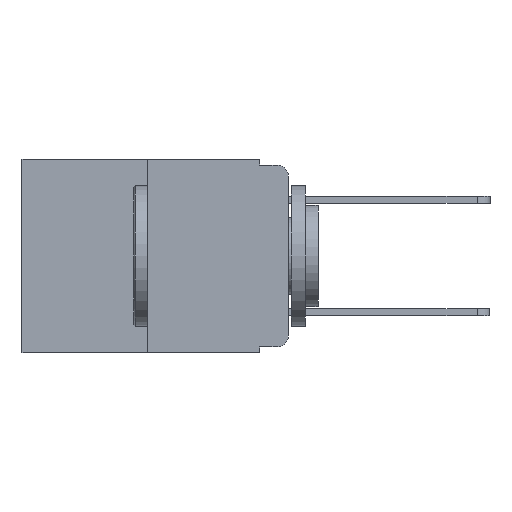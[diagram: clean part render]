
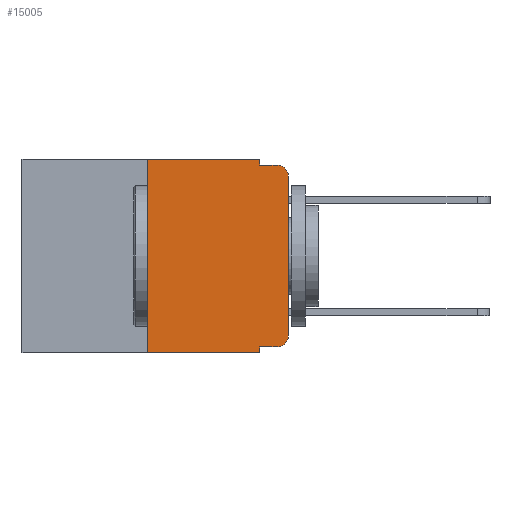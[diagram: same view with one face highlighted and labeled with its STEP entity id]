
A CAD part, left-side view. The second image highlights one B-rep face of the part: STEP entity #15005.
In plain terms, the highlighted planar face has unit normal (-1, 0, 0).
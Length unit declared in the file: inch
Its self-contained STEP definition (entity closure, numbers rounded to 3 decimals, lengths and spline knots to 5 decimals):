
#297 = LINE ( 'NONE', #2533, #17979 ) ;
#621 = EDGE_CURVE ( 'NONE', #21870, #22578, #9331, .T. ) ;
#885 = LINE ( 'NONE', #17494, #6171 ) ;
#1247 = DIRECTION ( 'NONE',  ( 0., 0., -1. ) ) ;
#1570 = AXIS2_PLACEMENT_3D ( 'NONE', #16847, #6264, #18528 ) ;
#1638 = DIRECTION ( 'NONE',  ( 0., 0., 1. ) ) ;
#1679 = DIRECTION ( 'NONE',  ( 0., 0., -1. ) ) ;
#1932 = LINE ( 'NONE', #11505, #19524 ) ;
#2103 = VERTEX_POINT ( 'NONE', #6217 ) ;
#2261 = VERTEX_POINT ( 'NONE', #13867 ) ;
#2464 = EDGE_CURVE ( 'NONE', #20631, #13815, #297, .T. ) ;
#2533 = CARTESIAN_POINT ( 'NONE',  ( 0., 0.473, -0.343 ) ) ;
#2588 = ORIENTED_EDGE ( 'NONE', *, *, #621, .T. ) ;
#2696 = ORIENTED_EDGE ( 'NONE', *, *, #2464, .T. ) ;
#2858 = DIRECTION ( 'NONE',  ( -1., 0., 0. ) ) ;
#2959 = ORIENTED_EDGE ( 'NONE', *, *, #13780, .F. ) ;
#3251 = DIRECTION ( 'NONE',  ( 0., -1., 0. ) ) ;
#4444 = PLANE ( 'NONE',  #1570 ) ;
#4547 = VECTOR ( 'NONE', #14518, 39.37008 ) ;
#4663 = LINE ( 'NONE', #22191, #22133 ) ;
#5026 = CARTESIAN_POINT ( 'NONE',  ( 0., 0.051, -0.333 ) ) ;
#5968 = CARTESIAN_POINT ( 'NONE',  ( 0., 0.051, -0.333 ) ) ;
#5973 = DIRECTION ( 'NONE',  ( 0., 0., 1. ) ) ;
#6171 = VECTOR ( 'NONE', #1638, 39.37008 ) ;
#6217 = CARTESIAN_POINT ( 'NONE',  ( 0., 0., -0.03 ) ) ;
#6264 = DIRECTION ( 'NONE',  ( 1., 0., 0. ) ) ;
#6957 = VERTEX_POINT ( 'NONE', #19107 ) ;
#7010 = EDGE_CURVE ( 'NONE', #18265, #2103, #885, .T. ) ;
#8526 = ORIENTED_EDGE ( 'NONE', *, *, #9167, .T. ) ;
#8953 = VECTOR ( 'NONE', #5973, 39.37008 ) ;
#9118 = EDGE_CURVE ( 'NONE', #2261, #10085, #17697, .T. ) ;
#9167 = EDGE_CURVE ( 'NONE', #22578, #18265, #15588, .T. ) ;
#9331 = LINE ( 'NONE', #5968, #4547 ) ;
#9724 = CARTESIAN_POINT ( 'NONE',  ( 0., 0.25, 0. ) ) ;
#10085 = VERTEX_POINT ( 'NONE', #18231 ) ;
#10205 = CARTESIAN_POINT ( 'NONE',  ( 0., 0.25, -0.343 ) ) ;
#10801 = EDGE_LOOP ( 'NONE', ( #19407, #13546, #22301, #21328, #12629, #13531, #2696, #2959, #2588, #8526 ) ) ;
#11505 = CARTESIAN_POINT ( 'NONE',  ( 0., 0.051, 0. ) ) ;
#11965 = CARTESIAN_POINT ( 'NONE',  ( 0., 0.051, -0.343 ) ) ;
#12397 = EDGE_CURVE ( 'NONE', #20631, #18599, #13690, .T. ) ;
#12404 = DIRECTION ( 'NONE',  ( -1., 0., 0. ) ) ;
#12629 = ORIENTED_EDGE ( 'NONE', *, *, #22168, .F. ) ;
#13531 = ORIENTED_EDGE ( 'NONE', *, *, #12397, .F. ) ;
#13537 = CARTESIAN_POINT ( 'NONE',  ( 0., 0.02, -0.03 ) ) ;
#13546 = ORIENTED_EDGE ( 'NONE', *, *, #16905, .T. ) ;
#13690 = LINE ( 'NONE', #21597, #8953 ) ;
#13780 = EDGE_CURVE ( 'NONE', #21870, #13815, #4663, .T. ) ;
#13815 = VERTEX_POINT ( 'NONE', #11965 ) ;
#13867 = CARTESIAN_POINT ( 'NONE',  ( 0., 0.051, -0.01 ) ) ;
#13884 = CARTESIAN_POINT ( 'NONE',  ( 0., 0.473, 0. ) ) ;
#14330 = CIRCLE ( 'NONE', #20142, 0.02 ) ;
#14518 = DIRECTION ( 'NONE',  ( 0., -1., 0. ) ) ;
#15005 = ADVANCED_FACE ( 'NONE', ( #22117 ), #4444, .F. ) ;
#15299 = DIRECTION ( 'NONE',  ( 0., 0., -1. ) ) ;
#15588 = CIRCLE ( 'NONE', #22434, 0.02 ) ;
#15700 = CARTESIAN_POINT ( 'NONE',  ( 0., 0.051, -0.01 ) ) ;
#16659 = CARTESIAN_POINT ( 'NONE',  ( 0., 0.02, -0.333 ) ) ;
#16847 = CARTESIAN_POINT ( 'NONE',  ( 0., 0.473, 0. ) ) ;
#16905 = EDGE_CURVE ( 'NONE', #2103, #10085, #14330, .T. ) ;
#17377 = CARTESIAN_POINT ( 'NONE',  ( 0., 0., -0.313 ) ) ;
#17494 = CARTESIAN_POINT ( 'NONE',  ( 0., 0., 0. ) ) ;
#17697 = LINE ( 'NONE', #15700, #21149 ) ;
#17753 = DIRECTION ( 'NONE',  ( 0., -1., 0. ) ) ;
#17979 = VECTOR ( 'NONE', #17753, 39.37008 ) ;
#18231 = CARTESIAN_POINT ( 'NONE',  ( 0., 0.02, -0.01 ) ) ;
#18265 = VERTEX_POINT ( 'NONE', #17377 ) ;
#18528 = DIRECTION ( 'NONE',  ( 0., 0., -1. ) ) ;
#18599 = VERTEX_POINT ( 'NONE', #9724 ) ;
#19019 = DIRECTION ( 'NONE',  ( 0., -1., 0. ) ) ;
#19107 = CARTESIAN_POINT ( 'NONE',  ( 0., 0.051, 0. ) ) ;
#19407 = ORIENTED_EDGE ( 'NONE', *, *, #7010, .T. ) ;
#19524 = VECTOR ( 'NONE', #21785, 39.37008 ) ;
#20142 = AXIS2_PLACEMENT_3D ( 'NONE', #13537, #2858, #15299 ) ;
#20267 = VECTOR ( 'NONE', #19019, 39.37008 ) ;
#20631 = VERTEX_POINT ( 'NONE', #10205 ) ;
#20806 = LINE ( 'NONE', #13884, #20267 ) ;
#21149 = VECTOR ( 'NONE', #3251, 39.37008 ) ;
#21160 = EDGE_CURVE ( 'NONE', #6957, #2261, #1932, .T. ) ;
#21328 = ORIENTED_EDGE ( 'NONE', *, *, #21160, .F. ) ;
#21597 = CARTESIAN_POINT ( 'NONE',  ( 0., 0.25, 0. ) ) ;
#21785 = DIRECTION ( 'NONE',  ( 0., 0., -1. ) ) ;
#21870 = VERTEX_POINT ( 'NONE', #5026 ) ;
#22117 = FACE_OUTER_BOUND ( 'NONE', #10801, .T. ) ;
#22133 = VECTOR ( 'NONE', #1247, 39.37008 ) ;
#22168 = EDGE_CURVE ( 'NONE', #18599, #6957, #20806, .T. ) ;
#22191 = CARTESIAN_POINT ( 'NONE',  ( 0., 0.051, 0. ) ) ;
#22301 = ORIENTED_EDGE ( 'NONE', *, *, #9118, .F. ) ;
#22434 = AXIS2_PLACEMENT_3D ( 'NONE', #22610, #12404, #1679 ) ;
#22578 = VERTEX_POINT ( 'NONE', #16659 ) ;
#22610 = CARTESIAN_POINT ( 'NONE',  ( 0., 0.02, -0.313 ) ) ;
